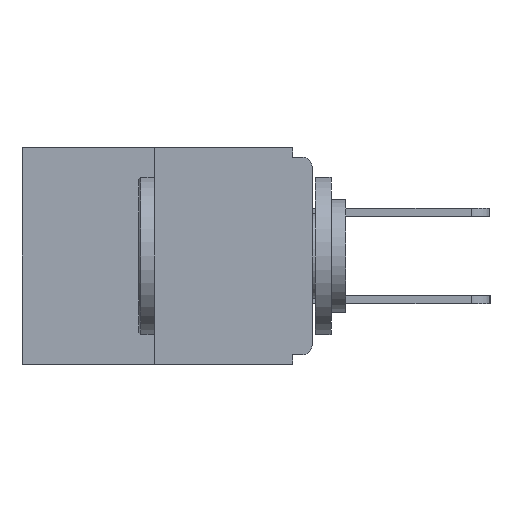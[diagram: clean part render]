
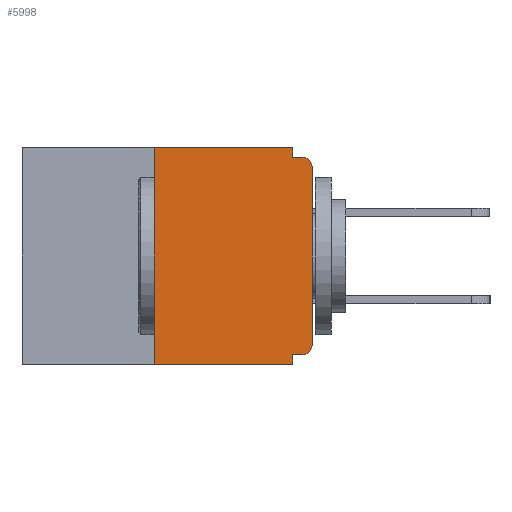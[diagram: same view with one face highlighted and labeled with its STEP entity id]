
A CAD part, left-side view. The second image highlights one B-rep face of the part: STEP entity #5998.
In plain terms, the highlighted planar face has unit normal (-1, 0, 0).
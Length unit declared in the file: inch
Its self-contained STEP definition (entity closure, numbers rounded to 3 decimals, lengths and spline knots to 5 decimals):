
#207 = VERTEX_POINT ( 'NONE', #14640 ) ;
#593 = DIRECTION ( 'NONE',  ( 0., -1., 0. ) ) ;
#1250 = CARTESIAN_POINT ( 'NONE',  ( 0., 0., -0.328 ) ) ;
#1353 = VECTOR ( 'NONE', #18939, 39.37008 ) ;
#1732 = VERTEX_POINT ( 'NONE', #10509 ) ;
#1914 = CARTESIAN_POINT ( 'NONE',  ( 0., 0., -0.03 ) ) ;
#1991 = DIRECTION ( 'NONE',  ( 0., -1., 0. ) ) ;
#2198 = VECTOR ( 'NONE', #19598, 39.37008 ) ;
#3026 = VECTOR ( 'NONE', #8125, 39.37008 ) ;
#3507 = LINE ( 'NONE', #4808, #5323 ) ;
#3626 = CARTESIAN_POINT ( 'NONE',  ( 0., 0.031, -0.343 ) ) ;
#4407 = ORIENTED_EDGE ( 'NONE', *, *, #15895, .F. ) ;
#4752 = CARTESIAN_POINT ( 'NONE',  ( 0., 0.46, -0.343 ) ) ;
#4791 = ORIENTED_EDGE ( 'NONE', *, *, #16582, .F. ) ;
#4808 = CARTESIAN_POINT ( 'NONE',  ( 0., 0.031, -0.343 ) ) ;
#5018 = VERTEX_POINT ( 'NONE', #14523 ) ;
#5029 = AXIS2_PLACEMENT_3D ( 'NONE', #5432, #6882, #13576 ) ;
#5323 = VECTOR ( 'NONE', #18256, 39.37008 ) ;
#5432 = CARTESIAN_POINT ( 'NONE',  ( 0., 0.46, 0. ) ) ;
#5516 = CIRCLE ( 'NONE', #10629, 0.015 ) ;
#5998 = ADVANCED_FACE ( 'NONE', ( #17139 ), #7017, .F. ) ;
#6131 = EDGE_CURVE ( 'NONE', #10774, #10799, #12702, .T. ) ;
#6410 = CARTESIAN_POINT ( 'NONE',  ( 0., 0.031, -0.328 ) ) ;
#6436 = VERTEX_POINT ( 'NONE', #18880 ) ;
#6515 = CARTESIAN_POINT ( 'NONE',  ( 0., 0., -0.015 ) ) ;
#6882 = DIRECTION ( 'NONE',  ( 1., 0., 0. ) ) ;
#6924 = LINE ( 'NONE', #1250, #3026 ) ;
#7017 = PLANE ( 'NONE',  #5029 ) ;
#7204 = ORIENTED_EDGE ( 'NONE', *, *, #6131, .T. ) ;
#7809 = EDGE_CURVE ( 'NONE', #6436, #14406, #13921, .T. ) ;
#8125 = DIRECTION ( 'NONE',  ( 0., 1., 0. ) ) ;
#8146 = EDGE_CURVE ( 'NONE', #1732, #10774, #16227, .T. ) ;
#8323 = EDGE_CURVE ( 'NONE', #14795, #10799, #15984, .T. ) ;
#8876 = VERTEX_POINT ( 'NONE', #6410 ) ;
#8959 = LINE ( 'NONE', #12091, #13394 ) ;
#8999 = EDGE_CURVE ( 'NONE', #8876, #14406, #3507, .T. ) ;
#9293 = DIRECTION ( 'NONE',  ( -1., 0., 0. ) ) ;
#9867 = CARTESIAN_POINT ( 'NONE',  ( 0., 0., 0. ) ) ;
#10509 = CARTESIAN_POINT ( 'NONE',  ( 0., 0., -0.313 ) ) ;
#10629 = AXIS2_PLACEMENT_3D ( 'NONE', #12721, #9293, #14338 ) ;
#10774 = VERTEX_POINT ( 'NONE', #1914 ) ;
#10799 = VERTEX_POINT ( 'NONE', #16977 ) ;
#10812 = ORIENTED_EDGE ( 'NONE', *, *, #8999, .F. ) ;
#11254 = VECTOR ( 'NONE', #13566, 39.37008 ) ;
#11426 = DIRECTION ( 'NONE',  ( -1., 0., 0. ) ) ;
#12090 = ORIENTED_EDGE ( 'NONE', *, *, #18179, .F. ) ;
#12091 = CARTESIAN_POINT ( 'NONE',  ( 0., 0.46, 0. ) ) ;
#12299 = LINE ( 'NONE', #18371, #11254 ) ;
#12702 = CIRCLE ( 'NONE', #16589, 0.015 ) ;
#12721 = CARTESIAN_POINT ( 'NONE',  ( 0., 0.015, -0.313 ) ) ;
#13394 = VECTOR ( 'NONE', #593, 39.37008 ) ;
#13566 = DIRECTION ( 'NONE',  ( 0., 0., -1. ) ) ;
#13576 = DIRECTION ( 'NONE',  ( 0., 0., -1. ) ) ;
#13921 = LINE ( 'NONE', #4752, #17314 ) ;
#13990 = CARTESIAN_POINT ( 'NONE',  ( 0., 0.25, 0. ) ) ;
#14338 = DIRECTION ( 'NONE',  ( 0., 0., -1. ) ) ;
#14406 = VERTEX_POINT ( 'NONE', #3626 ) ;
#14523 = CARTESIAN_POINT ( 'NONE',  ( 0., 0.015, -0.328 ) ) ;
#14640 = CARTESIAN_POINT ( 'NONE',  ( 0., 0.031, 0. ) ) ;
#14783 = DIRECTION ( 'NONE',  ( 0., 0., -1. ) ) ;
#14795 = VERTEX_POINT ( 'NONE', #17844 ) ;
#14923 = ORIENTED_EDGE ( 'NONE', *, *, #17832, .F. ) ;
#15158 = EDGE_LOOP ( 'NONE', ( #4791, #12090, #16255, #10812, #4407, #21051, #17560, #7204, #18482, #14923 ) ) ;
#15247 = EDGE_CURVE ( 'NONE', #5018, #1732, #5516, .T. ) ;
#15895 = EDGE_CURVE ( 'NONE', #5018, #8876, #6924, .T. ) ;
#15984 = LINE ( 'NONE', #6515, #2198 ) ;
#16227 = LINE ( 'NONE', #9867, #19594 ) ;
#16247 = CARTESIAN_POINT ( 'NONE',  ( 0., 0.015, -0.03 ) ) ;
#16255 = ORIENTED_EDGE ( 'NONE', *, *, #7809, .T. ) ;
#16582 = EDGE_CURVE ( 'NONE', #19659, #207, #8959, .T. ) ;
#16589 = AXIS2_PLACEMENT_3D ( 'NONE', #16247, #11426, #14783 ) ;
#16977 = CARTESIAN_POINT ( 'NONE',  ( 0., 0.015, -0.015 ) ) ;
#17139 = FACE_OUTER_BOUND ( 'NONE', #15158, .T. ) ;
#17314 = VECTOR ( 'NONE', #1991, 39.37008 ) ;
#17560 = ORIENTED_EDGE ( 'NONE', *, *, #8146, .T. ) ;
#17832 = EDGE_CURVE ( 'NONE', #207, #14795, #12299, .T. ) ;
#17844 = CARTESIAN_POINT ( 'NONE',  ( 0., 0.031, -0.015 ) ) ;
#18179 = EDGE_CURVE ( 'NONE', #6436, #19659, #20098, .T. ) ;
#18256 = DIRECTION ( 'NONE',  ( 0., 0., -1. ) ) ;
#18371 = CARTESIAN_POINT ( 'NONE',  ( 0., 0.031, 0. ) ) ;
#18471 = DIRECTION ( 'NONE',  ( 0., 0., 1. ) ) ;
#18482 = ORIENTED_EDGE ( 'NONE', *, *, #8323, .F. ) ;
#18880 = CARTESIAN_POINT ( 'NONE',  ( 0., 0.25, -0.343 ) ) ;
#18939 = DIRECTION ( 'NONE',  ( 0., 0., 1. ) ) ;
#19220 = CARTESIAN_POINT ( 'NONE',  ( 0., 0.25, 0. ) ) ;
#19594 = VECTOR ( 'NONE', #18471, 39.37008 ) ;
#19598 = DIRECTION ( 'NONE',  ( 0., -1., 0. ) ) ;
#19659 = VERTEX_POINT ( 'NONE', #19220 ) ;
#20098 = LINE ( 'NONE', #13990, #1353 ) ;
#21051 = ORIENTED_EDGE ( 'NONE', *, *, #15247, .T. ) ;
